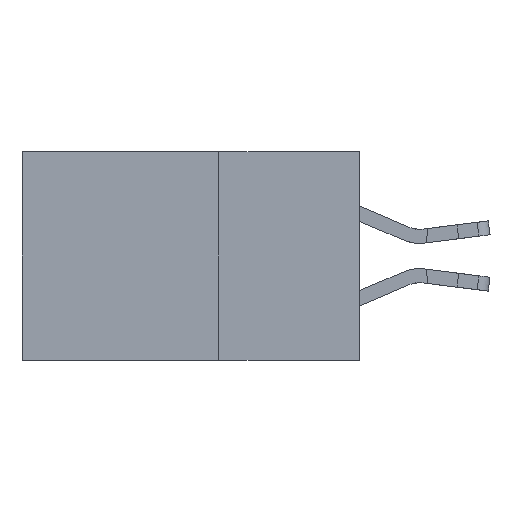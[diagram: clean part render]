
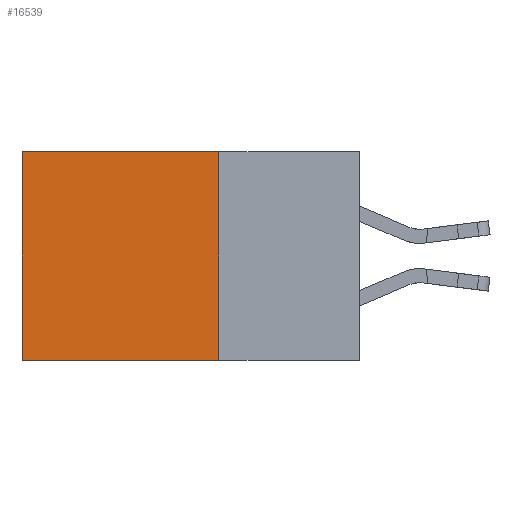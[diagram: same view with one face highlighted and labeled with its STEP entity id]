
A CAD part, left-side view. The second image highlights one B-rep face of the part: STEP entity #16539.
In plain terms, the highlighted planar face has unit normal (-1, 0, 0).
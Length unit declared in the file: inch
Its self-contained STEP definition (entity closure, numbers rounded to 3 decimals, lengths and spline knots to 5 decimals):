
#876 = VECTOR ( 'NONE', #3379, 39.37008 ) ;
#1202 = CARTESIAN_POINT ( 'NONE',  ( 0.2875, 0.25, -0.37 ) ) ;
#1491 = DIRECTION ( 'NONE',  ( 0., 0., -1. ) ) ;
#1580 = DIRECTION ( 'NONE',  ( 1., 0., 0. ) ) ;
#2658 = EDGE_CURVE ( 'NONE', #19139, #20686, #16003, .T. ) ;
#3379 = DIRECTION ( 'NONE',  ( 0., 1., 0. ) ) ;
#4756 = ORIENTED_EDGE ( 'NONE', *, *, #18402, .F. ) ;
#6612 = LINE ( 'NONE', #1202, #876 ) ;
#6915 = VECTOR ( 'NONE', #1491, 39.37008 ) ;
#9129 = EDGE_LOOP ( 'NONE', ( #19501, #4756, #10108, #20072 ) ) ;
#10108 = ORIENTED_EDGE ( 'NONE', *, *, #23894, .F. ) ;
#10373 = CARTESIAN_POINT ( 'NONE',  ( 0.2875, 0.25, 0. ) ) ;
#11876 = VERTEX_POINT ( 'NONE', #20218 ) ;
#13455 = LINE ( 'NONE', #10373, #14085 ) ;
#14085 = VECTOR ( 'NONE', #24584, 39.37008 ) ;
#14162 = CARTESIAN_POINT ( 'NONE',  ( 0.2875, 0.25, 0. ) ) ;
#14431 = FACE_OUTER_BOUND ( 'NONE', #9129, .T. ) ;
#15750 = CARTESIAN_POINT ( 'NONE',  ( 0.2875, 0.25, -0.37 ) ) ;
#16003 = LINE ( 'NONE', #21755, #26149 ) ;
#16217 = DIRECTION ( 'NONE',  ( 0., 0., -1. ) ) ;
#16539 = ADVANCED_FACE ( 'NONE', ( #14431 ), #22243, .F. ) ;
#17097 = VERTEX_POINT ( 'NONE', #15750 ) ;
#18402 = EDGE_CURVE ( 'NONE', #17097, #11876, #6612, .T. ) ;
#18481 = LINE ( 'NONE', #26239, #6915 ) ;
#18742 = AXIS2_PLACEMENT_3D ( 'NONE', #14162, #1580, #16217 ) ;
#19139 = VERTEX_POINT ( 'NONE', #23631 ) ;
#19501 = ORIENTED_EDGE ( 'NONE', *, *, #25006, .T. ) ;
#20072 = ORIENTED_EDGE ( 'NONE', *, *, #2658, .T. ) ;
#20218 = CARTESIAN_POINT ( 'NONE',  ( 0.2875, 0.6, -0.37 ) ) ;
#20686 = VERTEX_POINT ( 'NONE', #26127 ) ;
#21755 = CARTESIAN_POINT ( 'NONE',  ( 0.2875, 0.25, 0. ) ) ;
#22198 = DIRECTION ( 'NONE',  ( 0., 1., 0. ) ) ;
#22243 = PLANE ( 'NONE',  #18742 ) ;
#23631 = CARTESIAN_POINT ( 'NONE',  ( 0.2875, 0.25, 0. ) ) ;
#23894 = EDGE_CURVE ( 'NONE', #19139, #17097, #13455, .T. ) ;
#24584 = DIRECTION ( 'NONE',  ( 0., 0., -1. ) ) ;
#25006 = EDGE_CURVE ( 'NONE', #20686, #11876, #18481, .T. ) ;
#26127 = CARTESIAN_POINT ( 'NONE',  ( 0.2875, 0.6, 0. ) ) ;
#26149 = VECTOR ( 'NONE', #22198, 39.37008 ) ;
#26239 = CARTESIAN_POINT ( 'NONE',  ( 0.2875, 0.6, 0. ) ) ;
